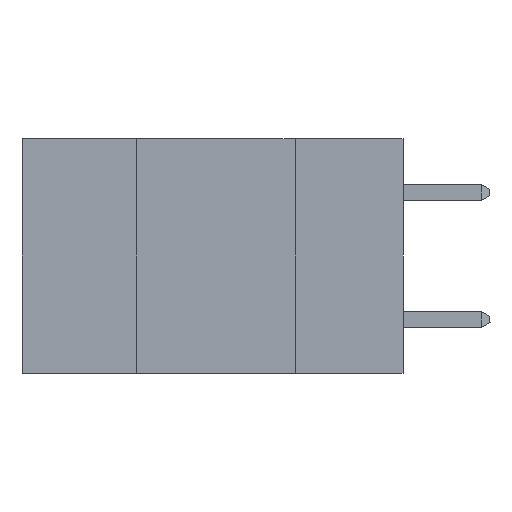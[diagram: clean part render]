
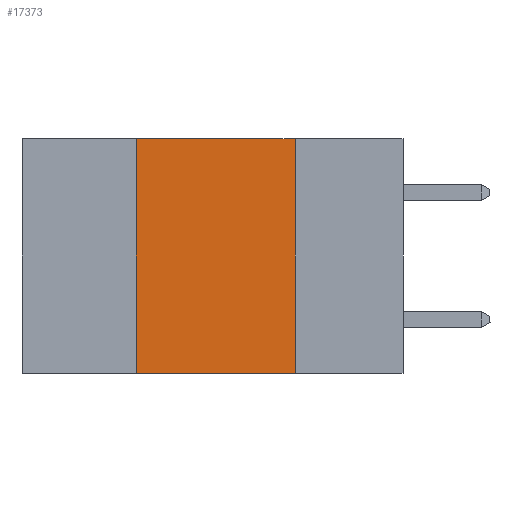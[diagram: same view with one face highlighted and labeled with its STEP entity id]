
A CAD part, left-side view. The second image highlights one B-rep face of the part: STEP entity #17373.
In plain terms, the highlighted planar face has unit normal (-1, 0, 0).
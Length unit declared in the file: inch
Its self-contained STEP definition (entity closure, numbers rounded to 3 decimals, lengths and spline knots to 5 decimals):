
#301 = FACE_OUTER_BOUND ( 'NONE', #4448, .T. ) ;
#430 = DIRECTION ( 'NONE',  ( 0., 0., -1. ) ) ;
#845 = DIRECTION ( 'NONE',  ( 0., -1., 0. ) ) ;
#1152 = CARTESIAN_POINT ( 'NONE',  ( 0., 0.17, 0. ) ) ;
#2639 = AXIS2_PLACEMENT_3D ( 'NONE', #15821, #23562, #430 ) ;
#2772 = CARTESIAN_POINT ( 'NONE',  ( 0., 0.42, 0. ) ) ;
#3057 = LINE ( 'NONE', #1152, #10092 ) ;
#3426 = EDGE_CURVE ( 'NONE', #8804, #24691, #7276, .T. ) ;
#4448 = EDGE_LOOP ( 'NONE', ( #15168, #23092, #20257, #14443 ) ) ;
#4760 = LINE ( 'NONE', #12894, #15467 ) ;
#7276 = LINE ( 'NONE', #24566, #10322 ) ;
#8057 = PLANE ( 'NONE',  #2639 ) ;
#8804 = VERTEX_POINT ( 'NONE', #25058 ) ;
#9059 = CARTESIAN_POINT ( 'NONE',  ( 0., 0.17, -0.37 ) ) ;
#9571 = DIRECTION ( 'NONE',  ( 0., -1., 0. ) ) ;
#10092 = VECTOR ( 'NONE', #22620, 39.37008 ) ;
#10322 = VECTOR ( 'NONE', #9571, 39.37008 ) ;
#12667 = CARTESIAN_POINT ( 'NONE',  ( 0., 0.6, 0. ) ) ;
#12695 = EDGE_CURVE ( 'NONE', #8804, #22115, #4760, .T. ) ;
#12894 = CARTESIAN_POINT ( 'NONE',  ( 0., 0.42, 0. ) ) ;
#13519 = VECTOR ( 'NONE', #845, 39.37008 ) ;
#14443 = ORIENTED_EDGE ( 'NONE', *, *, #3426, .T. ) ;
#15000 = VERTEX_POINT ( 'NONE', #22950 ) ;
#15168 = ORIENTED_EDGE ( 'NONE', *, *, #23451, .F. ) ;
#15467 = VECTOR ( 'NONE', #20393, 39.37008 ) ;
#15690 = EDGE_CURVE ( 'NONE', #22115, #15000, #16474, .T. ) ;
#15821 = CARTESIAN_POINT ( 'NONE',  ( 0., 0.6, 0. ) ) ;
#16474 = LINE ( 'NONE', #12667, #13519 ) ;
#17373 = ADVANCED_FACE ( 'NONE', ( #301 ), #8057, .F. ) ;
#20257 = ORIENTED_EDGE ( 'NONE', *, *, #12695, .F. ) ;
#20393 = DIRECTION ( 'NONE',  ( 0., 0., 1. ) ) ;
#22115 = VERTEX_POINT ( 'NONE', #2772 ) ;
#22620 = DIRECTION ( 'NONE',  ( 0., 0., -1. ) ) ;
#22950 = CARTESIAN_POINT ( 'NONE',  ( 0., 0.17, 0. ) ) ;
#23092 = ORIENTED_EDGE ( 'NONE', *, *, #15690, .F. ) ;
#23451 = EDGE_CURVE ( 'NONE', #15000, #24691, #3057, .T. ) ;
#23562 = DIRECTION ( 'NONE',  ( 1., 0., 0. ) ) ;
#24566 = CARTESIAN_POINT ( 'NONE',  ( 0., 0.6, -0.37 ) ) ;
#24691 = VERTEX_POINT ( 'NONE', #9059 ) ;
#25058 = CARTESIAN_POINT ( 'NONE',  ( 0., 0.42, -0.37 ) ) ;
